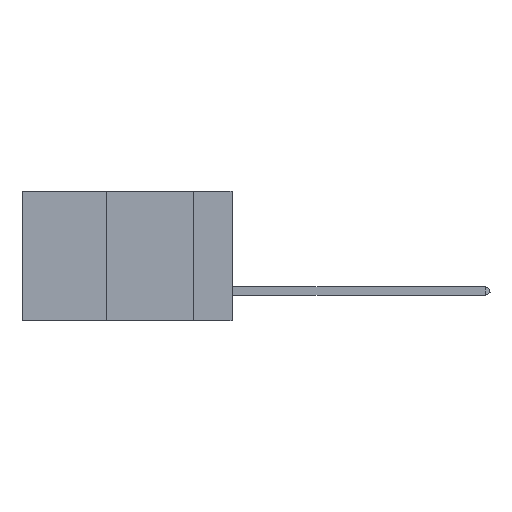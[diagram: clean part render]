
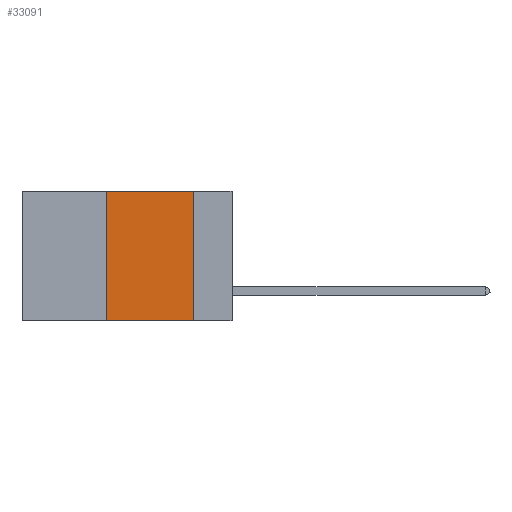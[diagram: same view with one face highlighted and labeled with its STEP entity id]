
A CAD part, left-side view. The second image highlights one B-rep face of the part: STEP entity #33091.
In plain terms, the highlighted planar face has unit normal (-1, 0, 0).
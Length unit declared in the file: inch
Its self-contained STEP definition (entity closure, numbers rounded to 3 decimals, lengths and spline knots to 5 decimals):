
#792 = CARTESIAN_POINT ( 'NONE',  ( 0., 0.6, 0. ) ) ;
#1073 = CARTESIAN_POINT ( 'NONE',  ( 0., 0.11, 0. ) ) ;
#1190 = FACE_OUTER_BOUND ( 'NONE', #23688, .T. ) ;
#1874 = ORIENTED_EDGE ( 'NONE', *, *, #6148, .F. ) ;
#5534 = CARTESIAN_POINT ( 'NONE',  ( 0., 0.36, 0. ) ) ;
#6148 = EDGE_CURVE ( 'NONE', #33595, #13335, #33524, .T. ) ;
#7543 = VECTOR ( 'NONE', #43162, 39.37008 ) ;
#7870 = PLANE ( 'NONE',  #30539 ) ;
#8390 = DIRECTION ( 'NONE',  ( 0., 0., 1. ) ) ;
#10494 = CARTESIAN_POINT ( 'NONE',  ( 0., 0.36, -0.37 ) ) ;
#12250 = DIRECTION ( 'NONE',  ( 0., -1., 0. ) ) ;
#13335 = VERTEX_POINT ( 'NONE', #1073 ) ;
#17993 = DIRECTION ( 'NONE',  ( 0., 0., -1. ) ) ;
#22202 = ORIENTED_EDGE ( 'NONE', *, *, #36740, .F. ) ;
#22492 = LINE ( 'NONE', #5534, #27936 ) ;
#23340 = EDGE_CURVE ( 'NONE', #13335, #43538, #24871, .T. ) ;
#23688 = EDGE_LOOP ( 'NONE', ( #28115, #1874, #22202, #30949 ) ) ;
#24602 = EDGE_CURVE ( 'NONE', #31205, #43538, #31335, .T. ) ;
#24871 = LINE ( 'NONE', #29833, #33019 ) ;
#27554 = VECTOR ( 'NONE', #12250, 39.37008 ) ;
#27936 = VECTOR ( 'NONE', #8390, 39.37008 ) ;
#28115 = ORIENTED_EDGE ( 'NONE', *, *, #23340, .F. ) ;
#28586 = DIRECTION ( 'NONE',  ( 0., 0., -1. ) ) ;
#29446 = CARTESIAN_POINT ( 'NONE',  ( 0., 0.6, 0. ) ) ;
#29833 = CARTESIAN_POINT ( 'NONE',  ( 0., 0.11, 0. ) ) ;
#30539 = AXIS2_PLACEMENT_3D ( 'NONE', #792, #42173, #17993 ) ;
#30949 = ORIENTED_EDGE ( 'NONE', *, *, #24602, .T. ) ;
#31205 = VERTEX_POINT ( 'NONE', #10494 ) ;
#31335 = LINE ( 'NONE', #36288, #27554 ) ;
#33012 = CARTESIAN_POINT ( 'NONE',  ( 0., 0.11, -0.37 ) ) ;
#33019 = VECTOR ( 'NONE', #28586, 39.37008 ) ;
#33091 = ADVANCED_FACE ( 'NONE', ( #1190 ), #7870, .F. ) ;
#33524 = LINE ( 'NONE', #29446, #7543 ) ;
#33595 = VERTEX_POINT ( 'NONE', #34163 ) ;
#34163 = CARTESIAN_POINT ( 'NONE',  ( 0., 0.36, 0. ) ) ;
#36288 = CARTESIAN_POINT ( 'NONE',  ( 0., 0.6, -0.37 ) ) ;
#36740 = EDGE_CURVE ( 'NONE', #31205, #33595, #22492, .T. ) ;
#42173 = DIRECTION ( 'NONE',  ( 1., 0., 0. ) ) ;
#43162 = DIRECTION ( 'NONE',  ( 0., -1., 0. ) ) ;
#43538 = VERTEX_POINT ( 'NONE', #33012 ) ;
